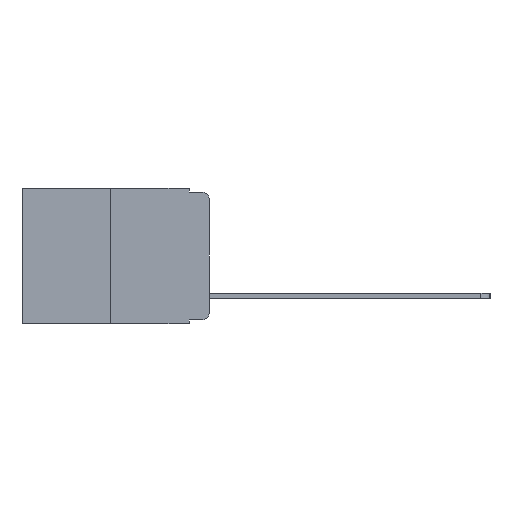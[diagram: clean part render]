
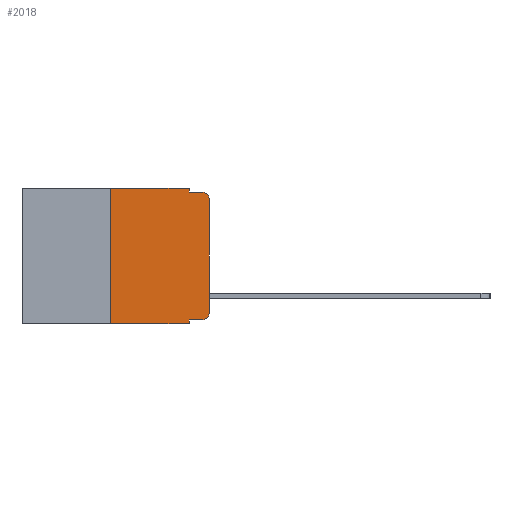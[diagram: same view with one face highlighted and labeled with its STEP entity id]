
A CAD part, left-side view. The second image highlights one B-rep face of the part: STEP entity #2018.
In plain terms, the highlighted planar face has unit normal (-1, 0, 0).
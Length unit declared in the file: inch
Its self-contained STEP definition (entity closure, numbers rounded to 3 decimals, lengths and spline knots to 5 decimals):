
#78 = DIRECTION ( 'NONE',  ( 0., -1., 0. ) ) ;
#426 = CARTESIAN_POINT ( 'NONE',  ( 0., 0.051, -0.01 ) ) ;
#874 = EDGE_CURVE ( 'NONE', #3874, #11962, #1771, .T. ) ;
#1041 = LINE ( 'NONE', #12485, #6050 ) ;
#1125 = CARTESIAN_POINT ( 'NONE',  ( 0., 0.473, 0. ) ) ;
#1617 = ORIENTED_EDGE ( 'NONE', *, *, #874, .T. ) ;
#1713 = CARTESIAN_POINT ( 'NONE',  ( 0., 0., -0.03 ) ) ;
#1737 = ORIENTED_EDGE ( 'NONE', *, *, #4782, .T. ) ;
#1771 = LINE ( 'NONE', #2785, #16061 ) ;
#1967 = EDGE_LOOP ( 'NONE', ( #2652, #6052, #17548, #10677, #9358, #3031, #1617, #12198, #9709, #1737 ) ) ;
#2018 = ADVANCED_FACE ( 'NONE', ( #16636 ), #8089, .F. ) ;
#2537 = CARTESIAN_POINT ( 'NONE',  ( 0., 0.02, -0.01 ) ) ;
#2652 = ORIENTED_EDGE ( 'NONE', *, *, #4987, .T. ) ;
#2785 = CARTESIAN_POINT ( 'NONE',  ( 0., 0.473, -0.343 ) ) ;
#2795 = LINE ( 'NONE', #10156, #7672 ) ;
#2913 = VECTOR ( 'NONE', #3648, 39.37008 ) ;
#3031 = ORIENTED_EDGE ( 'NONE', *, *, #14693, .F. ) ;
#3548 = CARTESIAN_POINT ( 'NONE',  ( 0., 0., 0. ) ) ;
#3648 = DIRECTION ( 'NONE',  ( 0., 0., -1. ) ) ;
#3814 = DIRECTION ( 'NONE',  ( 0., 0., -1. ) ) ;
#3844 = LINE ( 'NONE', #8219, #10954 ) ;
#3869 = CARTESIAN_POINT ( 'NONE',  ( 0., 0.25, 0. ) ) ;
#3874 = VERTEX_POINT ( 'NONE', #15481 ) ;
#4295 = CARTESIAN_POINT ( 'NONE',  ( 0., 0.02, -0.03 ) ) ;
#4782 = EDGE_CURVE ( 'NONE', #11969, #8251, #10487, .T. ) ;
#4838 = DIRECTION ( 'NONE',  ( 0., -1., 0. ) ) ;
#4851 = CARTESIAN_POINT ( 'NONE',  ( 0., 0.051, -0.343 ) ) ;
#4987 = EDGE_CURVE ( 'NONE', #8251, #18365, #6595, .T. ) ;
#6050 = VECTOR ( 'NONE', #7916, 39.37008 ) ;
#6052 = ORIENTED_EDGE ( 'NONE', *, *, #14851, .T. ) ;
#6163 = CARTESIAN_POINT ( 'NONE',  ( 0., 0.02, -0.313 ) ) ;
#6192 = EDGE_CURVE ( 'NONE', #17894, #13931, #1041, .T. ) ;
#6347 = LINE ( 'NONE', #7833, #2913 ) ;
#6501 = EDGE_CURVE ( 'NONE', #18335, #11969, #15799, .T. ) ;
#6595 = LINE ( 'NONE', #3548, #15498 ) ;
#6803 = CIRCLE ( 'NONE', #9504, 0.02 ) ;
#7637 = CARTESIAN_POINT ( 'NONE',  ( 0., 0.02, -0.333 ) ) ;
#7672 = VECTOR ( 'NONE', #12843, 39.37008 ) ;
#7726 = DIRECTION ( 'NONE',  ( 0., 0., 1. ) ) ;
#7833 = CARTESIAN_POINT ( 'NONE',  ( 0., 0.051, 0. ) ) ;
#7916 = DIRECTION ( 'NONE',  ( 0., -1., 0. ) ) ;
#8089 = PLANE ( 'NONE',  #15948 ) ;
#8219 = CARTESIAN_POINT ( 'NONE',  ( 0., 0.25, 0. ) ) ;
#8251 = VERTEX_POINT ( 'NONE', #9028 ) ;
#8777 = DIRECTION ( 'NONE',  ( -1., 0., 0. ) ) ;
#9028 = CARTESIAN_POINT ( 'NONE',  ( 0., 0., -0.313 ) ) ;
#9358 = ORIENTED_EDGE ( 'NONE', *, *, #6192, .F. ) ;
#9453 = CARTESIAN_POINT ( 'NONE',  ( 0., 0.051, -0.333 ) ) ;
#9504 = AXIS2_PLACEMENT_3D ( 'NONE', #4295, #8777, #10087 ) ;
#9709 = ORIENTED_EDGE ( 'NONE', *, *, #6501, .T. ) ;
#10087 = DIRECTION ( 'NONE',  ( 0., 0., -1. ) ) ;
#10156 = CARTESIAN_POINT ( 'NONE',  ( 0., 0.051, 0. ) ) ;
#10487 = CIRCLE ( 'NONE', #12547, 0.02 ) ;
#10677 = ORIENTED_EDGE ( 'NONE', *, *, #15326, .F. ) ;
#10954 = VECTOR ( 'NONE', #18220, 39.37008 ) ;
#11180 = DIRECTION ( 'NONE',  ( 1., 0., 0. ) ) ;
#11459 = LINE ( 'NONE', #15707, #16272 ) ;
#11803 = CARTESIAN_POINT ( 'NONE',  ( 0., 0.051, 0. ) ) ;
#11962 = VERTEX_POINT ( 'NONE', #4851 ) ;
#11969 = VERTEX_POINT ( 'NONE', #7637 ) ;
#12198 = ORIENTED_EDGE ( 'NONE', *, *, #14488, .F. ) ;
#12485 = CARTESIAN_POINT ( 'NONE',  ( 0., 0.473, 0. ) ) ;
#12547 = AXIS2_PLACEMENT_3D ( 'NONE', #6163, #17210, #12958 ) ;
#12843 = DIRECTION ( 'NONE',  ( 0., 0., -1. ) ) ;
#12958 = DIRECTION ( 'NONE',  ( 0., 0., -1. ) ) ;
#13320 = VERTEX_POINT ( 'NONE', #2537 ) ;
#13392 = DIRECTION ( 'NONE',  ( 0., -1., 0. ) ) ;
#13931 = VERTEX_POINT ( 'NONE', #11803 ) ;
#14488 = EDGE_CURVE ( 'NONE', #18335, #11962, #6347, .T. ) ;
#14519 = VERTEX_POINT ( 'NONE', #426 ) ;
#14693 = EDGE_CURVE ( 'NONE', #3874, #17894, #3844, .T. ) ;
#14851 = EDGE_CURVE ( 'NONE', #18365, #13320, #6803, .T. ) ;
#15326 = EDGE_CURVE ( 'NONE', #13931, #14519, #2795, .T. ) ;
#15373 = EDGE_CURVE ( 'NONE', #14519, #13320, #11459, .T. ) ;
#15481 = CARTESIAN_POINT ( 'NONE',  ( 0., 0.25, -0.343 ) ) ;
#15498 = VECTOR ( 'NONE', #7726, 39.37008 ) ;
#15707 = CARTESIAN_POINT ( 'NONE',  ( 0., 0.051, -0.01 ) ) ;
#15799 = LINE ( 'NONE', #17196, #15803 ) ;
#15803 = VECTOR ( 'NONE', #4838, 39.37008 ) ;
#15948 = AXIS2_PLACEMENT_3D ( 'NONE', #1125, #11180, #3814 ) ;
#16061 = VECTOR ( 'NONE', #78, 39.37008 ) ;
#16272 = VECTOR ( 'NONE', #13392, 39.37008 ) ;
#16636 = FACE_OUTER_BOUND ( 'NONE', #1967, .T. ) ;
#17196 = CARTESIAN_POINT ( 'NONE',  ( 0., 0.051, -0.333 ) ) ;
#17210 = DIRECTION ( 'NONE',  ( -1., 0., 0. ) ) ;
#17548 = ORIENTED_EDGE ( 'NONE', *, *, #15373, .F. ) ;
#17894 = VERTEX_POINT ( 'NONE', #3869 ) ;
#18220 = DIRECTION ( 'NONE',  ( 0., 0., 1. ) ) ;
#18335 = VERTEX_POINT ( 'NONE', #9453 ) ;
#18365 = VERTEX_POINT ( 'NONE', #1713 ) ;
